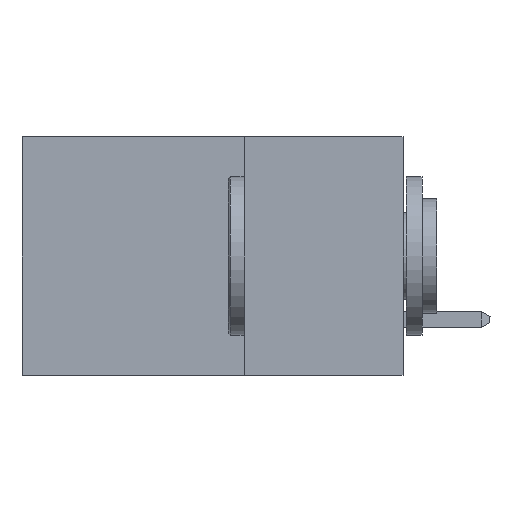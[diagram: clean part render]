
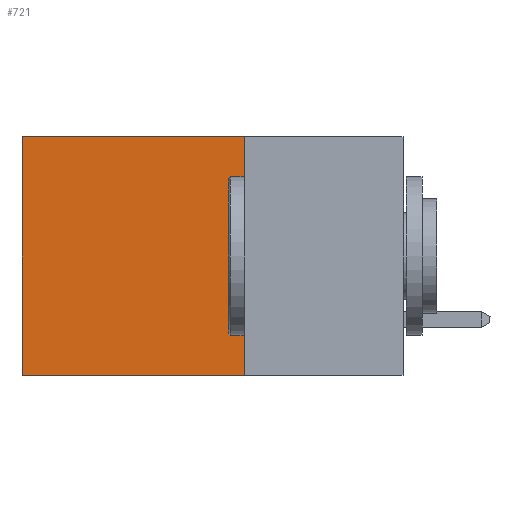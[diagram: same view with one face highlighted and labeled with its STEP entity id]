
A CAD part, left-side view. The second image highlights one B-rep face of the part: STEP entity #721.
In plain terms, the highlighted planar face has unit normal (-1, 0, 0).
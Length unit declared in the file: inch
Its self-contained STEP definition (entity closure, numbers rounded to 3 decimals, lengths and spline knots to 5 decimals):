
#115 = EDGE_CURVE ( 'NONE', #16607, #4058, #1579, .T. ) ;
#342 = ORIENTED_EDGE ( 'NONE', *, *, #2139, .T. ) ;
#677 = CARTESIAN_POINT ( 'NONE',  ( 0.2875, 0.25, 0. ) ) ;
#721 = ADVANCED_FACE ( 'NONE', ( #18222 ), #3979, .F. ) ;
#776 = VECTOR ( 'NONE', #5734, 39.37008 ) ;
#1280 = DIRECTION ( 'NONE',  ( 1., 0., 0. ) ) ;
#1579 = LINE ( 'NONE', #17920, #15991 ) ;
#2139 = EDGE_CURVE ( 'NONE', #16607, #5790, #9148, .T. ) ;
#3210 = LINE ( 'NONE', #4804, #13112 ) ;
#3912 = CARTESIAN_POINT ( 'NONE',  ( 0.2875, 0.25, -0.375 ) ) ;
#3979 = PLANE ( 'NONE',  #13732 ) ;
#4048 = DIRECTION ( 'NONE',  ( 0., 0., -1. ) ) ;
#4058 = VERTEX_POINT ( 'NONE', #17330 ) ;
#4414 = CARTESIAN_POINT ( 'NONE',  ( 0.2875, 0.6, 0. ) ) ;
#4804 = CARTESIAN_POINT ( 'NONE',  ( 0.2875, 0.6, -0.375 ) ) ;
#5121 = DIRECTION ( 'NONE',  ( 0., 0., -1. ) ) ;
#5734 = DIRECTION ( 'NONE',  ( 0., 1., 0. ) ) ;
#5790 = VERTEX_POINT ( 'NONE', #4414 ) ;
#6738 = CARTESIAN_POINT ( 'NONE',  ( 0.2875, 0.25, 0. ) ) ;
#6767 = ORIENTED_EDGE ( 'NONE', *, *, #18527, .T. ) ;
#9148 = LINE ( 'NONE', #6738, #15227 ) ;
#9505 = EDGE_LOOP ( 'NONE', ( #6767, #15255, #11572, #342 ) ) ;
#10468 = EDGE_CURVE ( 'NONE', #4058, #12479, #14512, .T. ) ;
#11572 = ORIENTED_EDGE ( 'NONE', *, *, #115, .F. ) ;
#11864 = DIRECTION ( 'NONE',  ( 0., 0., -1. ) ) ;
#12479 = VERTEX_POINT ( 'NONE', #18603 ) ;
#13112 = VECTOR ( 'NONE', #11864, 39.37008 ) ;
#13732 = AXIS2_PLACEMENT_3D ( 'NONE', #3912, #1280, #4048 ) ;
#14147 = DIRECTION ( 'NONE',  ( 0., 1., 0. ) ) ;
#14512 = LINE ( 'NONE', #17163, #776 ) ;
#15227 = VECTOR ( 'NONE', #14147, 39.37008 ) ;
#15255 = ORIENTED_EDGE ( 'NONE', *, *, #10468, .F. ) ;
#15991 = VECTOR ( 'NONE', #5121, 39.37008 ) ;
#16607 = VERTEX_POINT ( 'NONE', #677 ) ;
#17163 = CARTESIAN_POINT ( 'NONE',  ( 0.2875, 0.25, -0.375 ) ) ;
#17330 = CARTESIAN_POINT ( 'NONE',  ( 0.2875, 0.25, -0.375 ) ) ;
#17920 = CARTESIAN_POINT ( 'NONE',  ( 0.2875, 0.25, -0.375 ) ) ;
#18222 = FACE_OUTER_BOUND ( 'NONE', #9505, .T. ) ;
#18527 = EDGE_CURVE ( 'NONE', #5790, #12479, #3210, .T. ) ;
#18603 = CARTESIAN_POINT ( 'NONE',  ( 0.2875, 0.6, -0.375 ) ) ;
